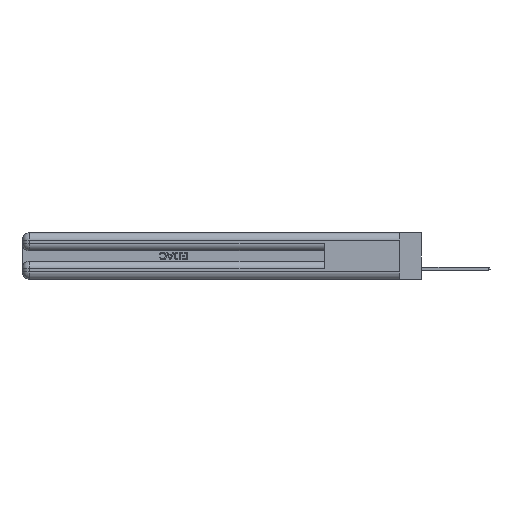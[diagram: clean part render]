
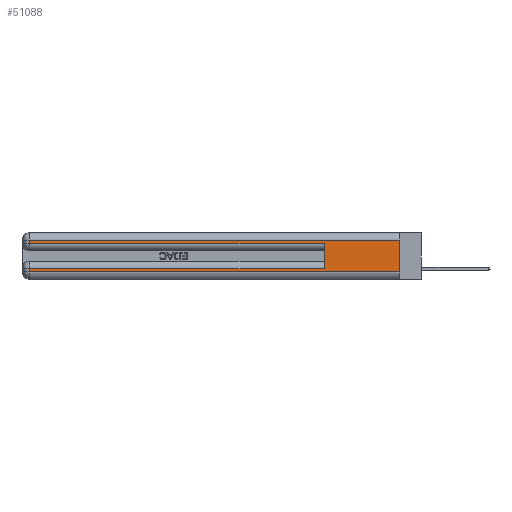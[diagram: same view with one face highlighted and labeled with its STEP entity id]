
A CAD part, left-side view. The second image highlights one B-rep face of the part: STEP entity #51088.
In plain terms, the highlighted planar face has unit normal (-1, 0, 0).
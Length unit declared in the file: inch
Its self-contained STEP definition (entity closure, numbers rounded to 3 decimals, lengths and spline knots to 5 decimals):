
#1078 = VECTOR ( 'NONE', #51833, 39.37008 ) ;
#1170 = VECTOR ( 'NONE', #20068, 39.37008 ) ;
#3446 = EDGE_CURVE ( 'NONE', #31738, #4513, #30433, .T. ) ;
#3653 = EDGE_LOOP ( 'NONE', ( #53331, #53280, #19457, #51432, #53970, #21358, #43245, #44120 ) ) ;
#4513 = VERTEX_POINT ( 'NONE', #53742 ) ;
#4957 = AXIS2_PLACEMENT_3D ( 'NONE', #48619, #19613, #37210 ) ;
#5375 = CARTESIAN_POINT ( 'NONE',  ( 0., 0., 0.085 ) ) ;
#6113 = CARTESIAN_POINT ( 'NONE',  ( 0., 0.6, 0.145 ) ) ;
#8092 = CARTESIAN_POINT ( 'NONE',  ( 0., 0., 0.31 ) ) ;
#8513 = VERTEX_POINT ( 'NONE', #50614 ) ;
#8889 = VERTEX_POINT ( 'NONE', #35235 ) ;
#10396 = DIRECTION ( 'NONE',  ( 0., 0., -1. ) ) ;
#10659 = VERTEX_POINT ( 'NONE', #52460 ) ;
#11972 = VECTOR ( 'NONE', #49695, 39.37008 ) ;
#12755 = DIRECTION ( 'NONE',  ( 0., 0., -1. ) ) ;
#12793 = CARTESIAN_POINT ( 'NONE',  ( 0., 2.94, 0.37 ) ) ;
#14089 = LINE ( 'NONE', #6113, #46600 ) ;
#14261 = VERTEX_POINT ( 'NONE', #26542 ) ;
#16557 = LINE ( 'NONE', #5375, #1078 ) ;
#17749 = EDGE_CURVE ( 'NONE', #31738, #14261, #37131, .T. ) ;
#18036 = CARTESIAN_POINT ( 'NONE',  ( 0., 0., 0.285 ) ) ;
#19118 = EDGE_CURVE ( 'NONE', #8513, #43623, #16557, .T. ) ;
#19457 = ORIENTED_EDGE ( 'NONE', *, *, #36039, .T. ) ;
#19613 = DIRECTION ( 'NONE',  ( 1., 0., 0. ) ) ;
#20068 = DIRECTION ( 'NONE',  ( 0., 0., -1. ) ) ;
#20254 = CARTESIAN_POINT ( 'NONE',  ( 0., 0., 0.37 ) ) ;
#21358 = ORIENTED_EDGE ( 'NONE', *, *, #19118, .T. ) ;
#21866 = EDGE_CURVE ( 'NONE', #43623, #8889, #35987, .T. ) ;
#21975 = CARTESIAN_POINT ( 'NONE',  ( 0., 2.94, 0.085 ) ) ;
#23401 = VECTOR ( 'NONE', #12755, 39.37008 ) ;
#26542 = CARTESIAN_POINT ( 'NONE',  ( 0., 0., 0.06 ) ) ;
#28290 = CARTESIAN_POINT ( 'NONE',  ( 0., 0., 0.31 ) ) ;
#29026 = LINE ( 'NONE', #18036, #50745 ) ;
#30433 = LINE ( 'NONE', #8092, #11972 ) ;
#30797 = FACE_OUTER_BOUND ( 'NONE', #3653, .T. ) ;
#31132 = CARTESIAN_POINT ( 'NONE',  ( 0., 2.94, 0.37 ) ) ;
#31201 = EDGE_CURVE ( 'NONE', #32900, #10659, #29026, .T. ) ;
#31738 = VERTEX_POINT ( 'NONE', #28290 ) ;
#32900 = VERTEX_POINT ( 'NONE', #44661 ) ;
#35235 = CARTESIAN_POINT ( 'NONE',  ( 0., 2.94, 0.06 ) ) ;
#35692 = DIRECTION ( 'NONE',  ( 0., 0., 1. ) ) ;
#35844 = PLANE ( 'NONE',  #4957 ) ;
#35987 = LINE ( 'NONE', #12793, #23401 ) ;
#36039 = EDGE_CURVE ( 'NONE', #4513, #32900, #53156, .T. ) ;
#37131 = LINE ( 'NONE', #20254, #1170 ) ;
#37159 = EDGE_CURVE ( 'NONE', #8889, #14261, #42976, .T. ) ;
#37210 = DIRECTION ( 'NONE',  ( 0., 0., -1. ) ) ;
#42976 = LINE ( 'NONE', #45137, #53701 ) ;
#43245 = ORIENTED_EDGE ( 'NONE', *, *, #21866, .T. ) ;
#43623 = VERTEX_POINT ( 'NONE', #21975 ) ;
#44120 = ORIENTED_EDGE ( 'NONE', *, *, #37159, .T. ) ;
#44661 = CARTESIAN_POINT ( 'NONE',  ( 0., 2.94, 0.285 ) ) ;
#45137 = CARTESIAN_POINT ( 'NONE',  ( 0., 0., 0.06 ) ) ;
#46600 = VECTOR ( 'NONE', #35692, 39.37008 ) ;
#48619 = CARTESIAN_POINT ( 'NONE',  ( 0., 0., 0.37 ) ) ;
#49695 = DIRECTION ( 'NONE',  ( 0., 1., 0. ) ) ;
#50523 = VECTOR ( 'NONE', #10396, 39.37008 ) ;
#50614 = CARTESIAN_POINT ( 'NONE',  ( 0., 0.6, 0.085 ) ) ;
#50745 = VECTOR ( 'NONE', #52098, 39.37008 ) ;
#51088 = ADVANCED_FACE ( 'NONE', ( #30797 ), #35844, .F. ) ;
#51432 = ORIENTED_EDGE ( 'NONE', *, *, #31201, .T. ) ;
#51833 = DIRECTION ( 'NONE',  ( 0., 1., 0. ) ) ;
#52098 = DIRECTION ( 'NONE',  ( 0., -1., 0. ) ) ;
#52266 = EDGE_CURVE ( 'NONE', #8513, #10659, #14089, .T. ) ;
#52460 = CARTESIAN_POINT ( 'NONE',  ( 0., 0.6, 0.285 ) ) ;
#53156 = LINE ( 'NONE', #31132, #50523 ) ;
#53280 = ORIENTED_EDGE ( 'NONE', *, *, #3446, .T. ) ;
#53331 = ORIENTED_EDGE ( 'NONE', *, *, #17749, .F. ) ;
#53701 = VECTOR ( 'NONE', #53745, 39.37008 ) ;
#53742 = CARTESIAN_POINT ( 'NONE',  ( 0., 2.94, 0.31 ) ) ;
#53745 = DIRECTION ( 'NONE',  ( 0., -1., 0. ) ) ;
#53970 = ORIENTED_EDGE ( 'NONE', *, *, #52266, .F. ) ;
